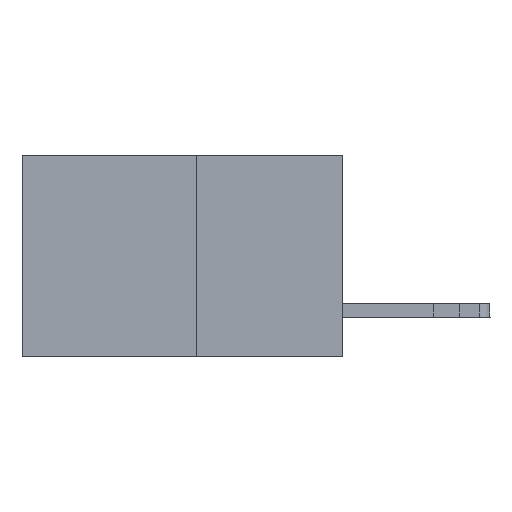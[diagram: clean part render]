
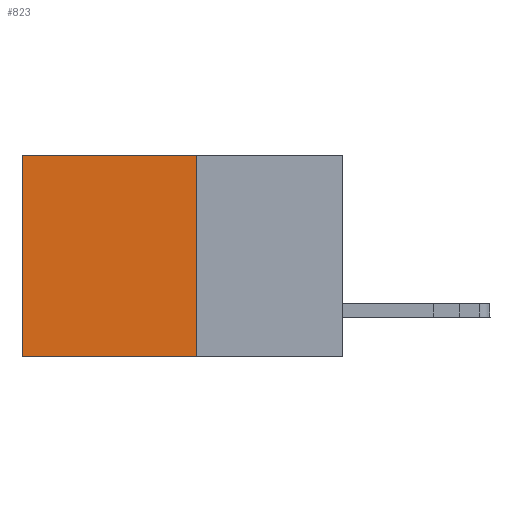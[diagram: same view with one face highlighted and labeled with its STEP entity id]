
A CAD part, left-side view. The second image highlights one B-rep face of the part: STEP entity #823.
In plain terms, the highlighted planar face has unit normal (-1, 0, 0).
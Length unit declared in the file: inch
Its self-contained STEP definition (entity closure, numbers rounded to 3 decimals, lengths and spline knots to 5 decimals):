
#89 = LINE ( 'NONE', #6194, #24700 ) ;
#603 = CARTESIAN_POINT ( 'NONE',  ( 0.277, 0.27, -0.37 ) ) ;
#823 = ADVANCED_FACE ( 'NONE', ( #1127 ), #25541, .F. ) ;
#924 = ORIENTED_EDGE ( 'NONE', *, *, #19579, .F. ) ;
#984 = VERTEX_POINT ( 'NONE', #19966 ) ;
#1127 = FACE_OUTER_BOUND ( 'NONE', #20334, .T. ) ;
#1534 = AXIS2_PLACEMENT_3D ( 'NONE', #11161, #7457, #21315 ) ;
#1834 = LINE ( 'NONE', #7401, #18797 ) ;
#1955 = CARTESIAN_POINT ( 'NONE',  ( 0.277, 0.59, -0.37 ) ) ;
#5945 = DIRECTION ( 'NONE',  ( 0., 1., 0. ) ) ;
#6194 = CARTESIAN_POINT ( 'NONE',  ( 0.277, 0.27, -0.37 ) ) ;
#6320 = EDGE_CURVE ( 'NONE', #984, #9467, #9524, .T. ) ;
#7401 = CARTESIAN_POINT ( 'NONE',  ( 0.277, 0.27, 0. ) ) ;
#7457 = DIRECTION ( 'NONE',  ( 1., 0., 0. ) ) ;
#8511 = VERTEX_POINT ( 'NONE', #23793 ) ;
#9467 = VERTEX_POINT ( 'NONE', #1955 ) ;
#9524 = LINE ( 'NONE', #21793, #11446 ) ;
#11161 = CARTESIAN_POINT ( 'NONE',  ( 0.277, 0.27, -0.37 ) ) ;
#11446 = VECTOR ( 'NONE', #25368, 39.37008 ) ;
#11970 = ORIENTED_EDGE ( 'NONE', *, *, #6320, .T. ) ;
#13845 = DIRECTION ( 'NONE',  ( 0., 0., -1. ) ) ;
#14217 = VERTEX_POINT ( 'NONE', #603 ) ;
#16951 = ORIENTED_EDGE ( 'NONE', *, *, #17469, .F. ) ;
#17469 = EDGE_CURVE ( 'NONE', #8511, #14217, #89, .T. ) ;
#18727 = ORIENTED_EDGE ( 'NONE', *, *, #21019, .T. ) ;
#18797 = VECTOR ( 'NONE', #25477, 39.37008 ) ;
#19579 = EDGE_CURVE ( 'NONE', #14217, #9467, #24293, .T. ) ;
#19966 = CARTESIAN_POINT ( 'NONE',  ( 0.277, 0.59, 0. ) ) ;
#20334 = EDGE_LOOP ( 'NONE', ( #11970, #924, #16951, #18727 ) ) ;
#21019 = EDGE_CURVE ( 'NONE', #8511, #984, #1834, .T. ) ;
#21315 = DIRECTION ( 'NONE',  ( 0., 0., -1. ) ) ;
#21793 = CARTESIAN_POINT ( 'NONE',  ( 0.277, 0.59, -0.37 ) ) ;
#22305 = CARTESIAN_POINT ( 'NONE',  ( 0.277, 0.27, -0.37 ) ) ;
#22939 = VECTOR ( 'NONE', #5945, 39.37008 ) ;
#23793 = CARTESIAN_POINT ( 'NONE',  ( 0.277, 0.27, 0. ) ) ;
#24293 = LINE ( 'NONE', #22305, #22939 ) ;
#24700 = VECTOR ( 'NONE', #13845, 39.37008 ) ;
#25368 = DIRECTION ( 'NONE',  ( 0., 0., -1. ) ) ;
#25477 = DIRECTION ( 'NONE',  ( 0., 1., 0. ) ) ;
#25541 = PLANE ( 'NONE',  #1534 ) ;
